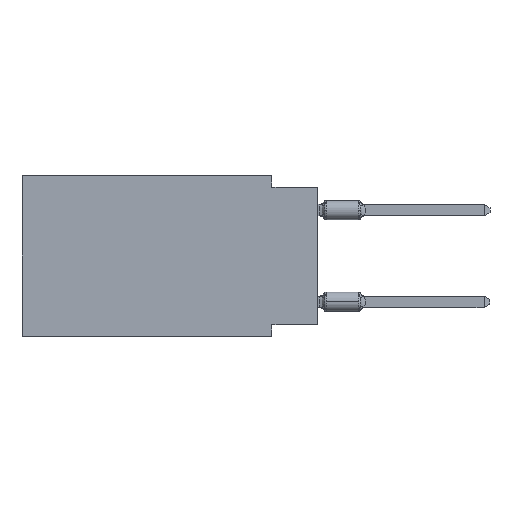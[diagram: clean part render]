
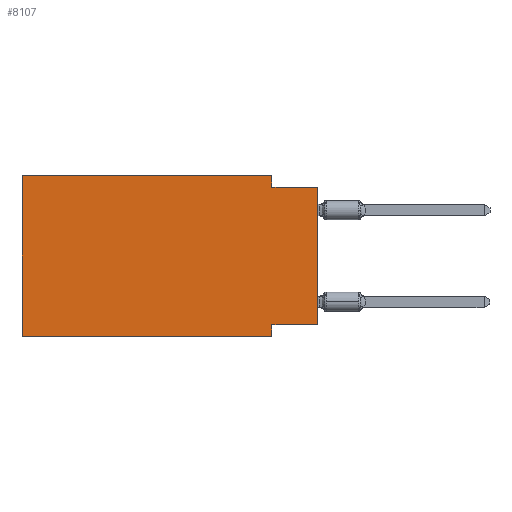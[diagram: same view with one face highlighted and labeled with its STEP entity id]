
A CAD part, left-side view. The second image highlights one B-rep face of the part: STEP entity #8107.
In plain terms, the highlighted planar face has unit normal (-1, 0, 0).
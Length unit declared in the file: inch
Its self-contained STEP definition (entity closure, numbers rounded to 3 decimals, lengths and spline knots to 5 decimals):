
#43 = CARTESIAN_POINT ( 'NONE',  ( 0., 0.1, -0.025 ) ) ;
#129 = VECTOR ( 'NONE', #2973, 39.37008 ) ;
#419 = VERTEX_POINT ( 'NONE', #12681 ) ;
#726 = VERTEX_POINT ( 'NONE', #43 ) ;
#955 = CARTESIAN_POINT ( 'NONE',  ( 0., 0.645, -0.35 ) ) ;
#1124 = CARTESIAN_POINT ( 'NONE',  ( 0., 0., -0.325 ) ) ;
#1165 = CARTESIAN_POINT ( 'NONE',  ( 0., 0.645, 0. ) ) ;
#1446 = EDGE_CURVE ( 'NONE', #2921, #12892, #10568, .T. ) ;
#1704 = PLANE ( 'NONE',  #6637 ) ;
#2049 = VERTEX_POINT ( 'NONE', #955 ) ;
#2272 = EDGE_LOOP ( 'NONE', ( #11935, #6348, #11841, #3202, #10715, #3267, #8391, #10826 ) ) ;
#2337 = CARTESIAN_POINT ( 'NONE',  ( 0., 0., -0.325 ) ) ;
#2743 = LINE ( 'NONE', #5988, #11232 ) ;
#2848 = CARTESIAN_POINT ( 'NONE',  ( 0., 0., -0.025 ) ) ;
#2904 = DIRECTION ( 'NONE',  ( 0., -1., 0. ) ) ;
#2921 = VERTEX_POINT ( 'NONE', #2337 ) ;
#2973 = DIRECTION ( 'NONE',  ( 0., 0., -1. ) ) ;
#3028 = VERTEX_POINT ( 'NONE', #7959 ) ;
#3043 = DIRECTION ( 'NONE',  ( 0., -1., 0. ) ) ;
#3099 = LINE ( 'NONE', #1165, #7292 ) ;
#3136 = CARTESIAN_POINT ( 'NONE',  ( 0., 0.1, 0. ) ) ;
#3202 = ORIENTED_EDGE ( 'NONE', *, *, #11305, .F. ) ;
#3267 = ORIENTED_EDGE ( 'NONE', *, *, #5038, .T. ) ;
#3433 = EDGE_CURVE ( 'NONE', #726, #3028, #12284, .T. ) ;
#3874 = EDGE_CURVE ( 'NONE', #12892, #419, #4073, .T. ) ;
#4073 = LINE ( 'NONE', #9375, #129 ) ;
#4227 = CARTESIAN_POINT ( 'NONE',  ( 0., 0.645, 0. ) ) ;
#4875 = DIRECTION ( 'NONE',  ( 1., 0., 0. ) ) ;
#4922 = DIRECTION ( 'NONE',  ( 0., 0., 1. ) ) ;
#5038 = EDGE_CURVE ( 'NONE', #2049, #419, #12341, .T. ) ;
#5611 = DIRECTION ( 'NONE',  ( 0., 1., 0. ) ) ;
#5928 = CARTESIAN_POINT ( 'NONE',  ( 0., 0.645, 0. ) ) ;
#5988 = CARTESIAN_POINT ( 'NONE',  ( 0., 0.1, 0. ) ) ;
#5991 = DIRECTION ( 'NONE',  ( 0., 0., -1. ) ) ;
#6311 = LINE ( 'NONE', #9396, #9983 ) ;
#6348 = ORIENTED_EDGE ( 'NONE', *, *, #3433, .F. ) ;
#6356 = LINE ( 'NONE', #12478, #6882 ) ;
#6444 = VERTEX_POINT ( 'NONE', #4227 ) ;
#6637 = AXIS2_PLACEMENT_3D ( 'NONE', #5928, #4875, #5991 ) ;
#6882 = VECTOR ( 'NONE', #3043, 39.37008 ) ;
#6898 = EDGE_CURVE ( 'NONE', #8730, #726, #2743, .T. ) ;
#7113 = CARTESIAN_POINT ( 'NONE',  ( 0., 0.645, -0.35 ) ) ;
#7292 = VECTOR ( 'NONE', #10679, 39.37008 ) ;
#7805 = EDGE_CURVE ( 'NONE', #2049, #6444, #3099, .T. ) ;
#7959 = CARTESIAN_POINT ( 'NONE',  ( 0., 0., -0.025 ) ) ;
#8107 = ADVANCED_FACE ( 'NONE', ( #11158 ), #1704, .F. ) ;
#8174 = DIRECTION ( 'NONE',  ( 0., 0., -1. ) ) ;
#8391 = ORIENTED_EDGE ( 'NONE', *, *, #3874, .F. ) ;
#8730 = VERTEX_POINT ( 'NONE', #3136 ) ;
#9375 = CARTESIAN_POINT ( 'NONE',  ( 0., 0.1, -0.35 ) ) ;
#9396 = CARTESIAN_POINT ( 'NONE',  ( 0., 0., 0. ) ) ;
#9673 = VECTOR ( 'NONE', #5611, 39.37008 ) ;
#9983 = VECTOR ( 'NONE', #4922, 39.37008 ) ;
#10568 = LINE ( 'NONE', #1124, #9673 ) ;
#10679 = DIRECTION ( 'NONE',  ( 0., 0., 1. ) ) ;
#10715 = ORIENTED_EDGE ( 'NONE', *, *, #7805, .F. ) ;
#10740 = VECTOR ( 'NONE', #2904, 39.37008 ) ;
#10826 = ORIENTED_EDGE ( 'NONE', *, *, #1446, .F. ) ;
#10945 = CARTESIAN_POINT ( 'NONE',  ( 0., 0.1, -0.325 ) ) ;
#11158 = FACE_OUTER_BOUND ( 'NONE', #2272, .T. ) ;
#11232 = VECTOR ( 'NONE', #8174, 39.37008 ) ;
#11261 = DIRECTION ( 'NONE',  ( 0., -1., 0. ) ) ;
#11305 = EDGE_CURVE ( 'NONE', #6444, #8730, #6356, .T. ) ;
#11841 = ORIENTED_EDGE ( 'NONE', *, *, #6898, .F. ) ;
#11935 = ORIENTED_EDGE ( 'NONE', *, *, #12477, .T. ) ;
#12284 = LINE ( 'NONE', #2848, #12632 ) ;
#12341 = LINE ( 'NONE', #7113, #10740 ) ;
#12477 = EDGE_CURVE ( 'NONE', #2921, #3028, #6311, .T. ) ;
#12478 = CARTESIAN_POINT ( 'NONE',  ( 0., 0.645, 0. ) ) ;
#12632 = VECTOR ( 'NONE', #11261, 39.37008 ) ;
#12681 = CARTESIAN_POINT ( 'NONE',  ( 0., 0.1, -0.35 ) ) ;
#12892 = VERTEX_POINT ( 'NONE', #10945 ) ;
